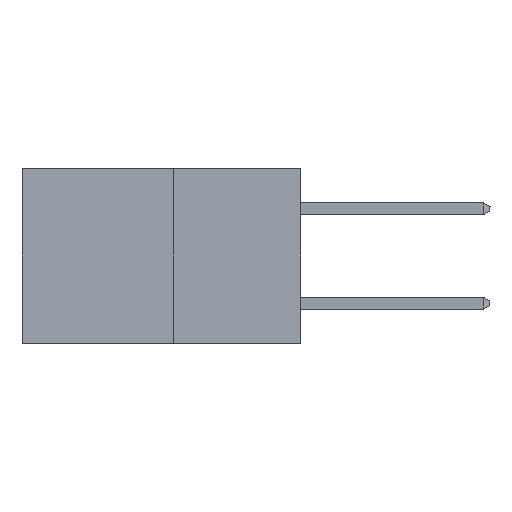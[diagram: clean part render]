
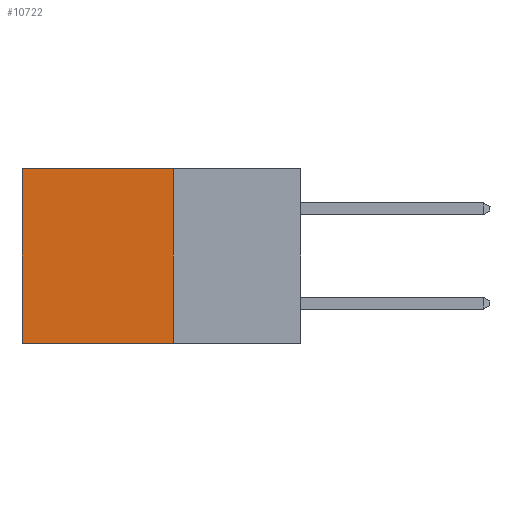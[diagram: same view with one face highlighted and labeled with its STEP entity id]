
A CAD part, left-side view. The second image highlights one B-rep face of the part: STEP entity #10722.
In plain terms, the highlighted planar face has unit normal (-1, 0, 0).
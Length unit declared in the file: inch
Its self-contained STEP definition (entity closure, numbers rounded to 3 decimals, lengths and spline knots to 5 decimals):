
#175 = DIRECTION ( 'NONE',  ( 0., 1., 0. ) ) ;
#221 = VECTOR ( 'NONE', #175, 39.37008 ) ;
#340 = DIRECTION ( 'NONE',  ( 0., 0., -1. ) ) ;
#849 = EDGE_CURVE ( 'NONE', #10845, #10260, #8141, .T. ) ;
#1141 = DIRECTION ( 'NONE',  ( 1., 0., 0. ) ) ;
#1233 = CARTESIAN_POINT ( 'NONE',  ( 0.277, 0.59, 0. ) ) ;
#1338 = CARTESIAN_POINT ( 'NONE',  ( 0.277, 0.27, 0. ) ) ;
#1546 = CARTESIAN_POINT ( 'NONE',  ( 0.277, 0.27, -0.37 ) ) ;
#2357 = ORIENTED_EDGE ( 'NONE', *, *, #5270, .T. ) ;
#2540 = DIRECTION ( 'NONE',  ( 0., 0., -1. ) ) ;
#3396 = ORIENTED_EDGE ( 'NONE', *, *, #9348, .T. ) ;
#3711 = CARTESIAN_POINT ( 'NONE',  ( 0.277, 0.59, -0.37 ) ) ;
#3853 = ORIENTED_EDGE ( 'NONE', *, *, #11707, .F. ) ;
#5270 = EDGE_CURVE ( 'NONE', #10845, #9208, #14153, .T. ) ;
#5339 = CARTESIAN_POINT ( 'NONE',  ( 0.277, 0.27, -0.37 ) ) ;
#5574 = PLANE ( 'NONE',  #9912 ) ;
#5939 = FACE_OUTER_BOUND ( 'NONE', #10786, .T. ) ;
#6061 = VECTOR ( 'NONE', #9368, 39.37008 ) ;
#6323 = VECTOR ( 'NONE', #340, 39.37008 ) ;
#6413 = LINE ( 'NONE', #12580, #6061 ) ;
#7642 = VERTEX_POINT ( 'NONE', #12775 ) ;
#8141 = LINE ( 'NONE', #5339, #11025 ) ;
#8893 = DIRECTION ( 'NONE',  ( 0., 0., -1. ) ) ;
#9208 = VERTEX_POINT ( 'NONE', #1233 ) ;
#9348 = EDGE_CURVE ( 'NONE', #9208, #7642, #12124, .T. ) ;
#9368 = DIRECTION ( 'NONE',  ( 0., 1., 0. ) ) ;
#9863 = ORIENTED_EDGE ( 'NONE', *, *, #849, .F. ) ;
#9912 = AXIS2_PLACEMENT_3D ( 'NONE', #13217, #1141, #8893 ) ;
#10260 = VERTEX_POINT ( 'NONE', #1546 ) ;
#10722 = ADVANCED_FACE ( 'NONE', ( #5939 ), #5574, .F. ) ;
#10786 = EDGE_LOOP ( 'NONE', ( #3396, #3853, #9863, #2357 ) ) ;
#10845 = VERTEX_POINT ( 'NONE', #1338 ) ;
#11025 = VECTOR ( 'NONE', #2540, 39.37008 ) ;
#11707 = EDGE_CURVE ( 'NONE', #10260, #7642, #6413, .T. ) ;
#12124 = LINE ( 'NONE', #3711, #6323 ) ;
#12580 = CARTESIAN_POINT ( 'NONE',  ( 0.277, 0.27, -0.37 ) ) ;
#12775 = CARTESIAN_POINT ( 'NONE',  ( 0.277, 0.59, -0.37 ) ) ;
#13217 = CARTESIAN_POINT ( 'NONE',  ( 0.277, 0.27, -0.37 ) ) ;
#13367 = CARTESIAN_POINT ( 'NONE',  ( 0.277, 0.27, 0. ) ) ;
#14153 = LINE ( 'NONE', #13367, #221 ) ;
